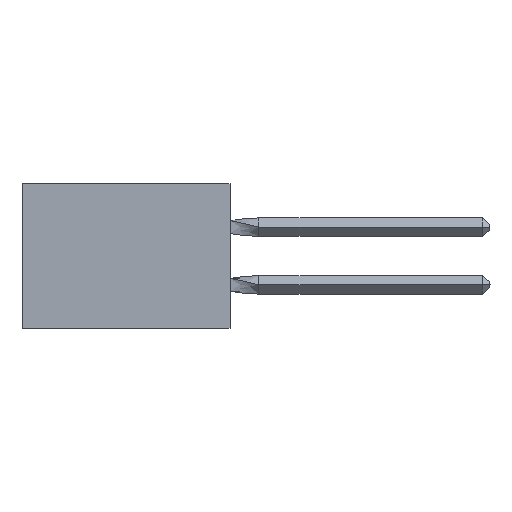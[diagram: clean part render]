
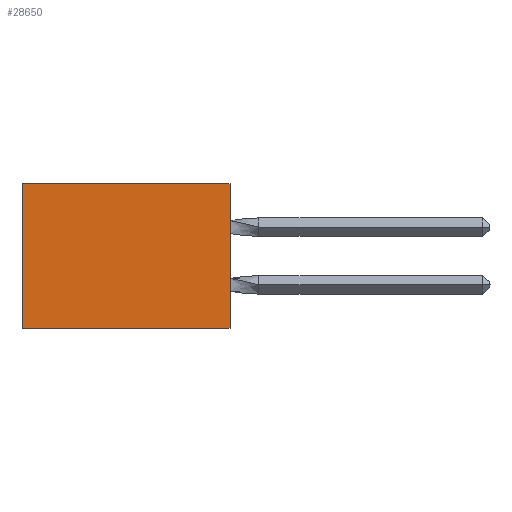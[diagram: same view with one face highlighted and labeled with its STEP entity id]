
A CAD part, left-side view. The second image highlights one B-rep face of the part: STEP entity #28650.
In plain terms, the highlighted planar face has unit normal (-1, 0, 0).
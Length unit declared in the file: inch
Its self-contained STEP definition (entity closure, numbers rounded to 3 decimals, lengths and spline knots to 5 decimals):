
#1717 = DIRECTION ( 'NONE',  ( 0., 0., -1. ) ) ;
#2243 = VERTEX_POINT ( 'NONE', #22399 ) ;
#3325 = FACE_OUTER_BOUND ( 'NONE', #24013, .T. ) ;
#3617 = DIRECTION ( 'NONE',  ( 0., 1., 0. ) ) ;
#7488 = CARTESIAN_POINT ( 'NONE',  ( 0.305, 0.72, 0. ) ) ;
#8642 = ORIENTED_EDGE ( 'NONE', *, *, #11522, .F. ) ;
#9768 = CARTESIAN_POINT ( 'NONE',  ( 0.305, 0., -0.5 ) ) ;
#10783 = DIRECTION ( 'NONE',  ( 0., 0., -1. ) ) ;
#11522 = EDGE_CURVE ( 'NONE', #2243, #32752, #19938, .T. ) ;
#13785 = VECTOR ( 'NONE', #28690, 39.37008 ) ;
#14025 = EDGE_CURVE ( 'NONE', #37685, #32752, #37899, .T. ) ;
#19022 = CARTESIAN_POINT ( 'NONE',  ( 0.305, 0., -0.5 ) ) ;
#19802 = DIRECTION ( 'NONE',  ( 0., 1., 0. ) ) ;
#19938 = LINE ( 'NONE', #19022, #22840 ) ;
#22052 = CARTESIAN_POINT ( 'NONE',  ( 0.305, 0.72, -0.5 ) ) ;
#22165 = ORIENTED_EDGE ( 'NONE', *, *, #38047, .T. ) ;
#22399 = CARTESIAN_POINT ( 'NONE',  ( 0.305, 0., -0.5 ) ) ;
#22832 = ORIENTED_EDGE ( 'NONE', *, *, #14025, .T. ) ;
#22840 = VECTOR ( 'NONE', #3617, 39.37008 ) ;
#23538 = PLANE ( 'NONE',  #28241 ) ;
#23675 = DIRECTION ( 'NONE',  ( 1., 0., 0. ) ) ;
#24013 = EDGE_LOOP ( 'NONE', ( #22832, #8642, #32874, #22165 ) ) ;
#25680 = VERTEX_POINT ( 'NONE', #35800 ) ;
#28241 = AXIS2_PLACEMENT_3D ( 'NONE', #39223, #23675, #1717 ) ;
#28650 = ADVANCED_FACE ( 'NONE', ( #3325 ), #23538, .F. ) ;
#28690 = DIRECTION ( 'NONE',  ( 0., 0., -1. ) ) ;
#32605 = CARTESIAN_POINT ( 'NONE',  ( 0.305, 0.72, -0.5 ) ) ;
#32752 = VERTEX_POINT ( 'NONE', #22052 ) ;
#32874 = ORIENTED_EDGE ( 'NONE', *, *, #33789, .F. ) ;
#33789 = EDGE_CURVE ( 'NONE', #25680, #2243, #39344, .T. ) ;
#34706 = LINE ( 'NONE', #38299, #40112 ) ;
#35800 = CARTESIAN_POINT ( 'NONE',  ( 0.305, 0., 0. ) ) ;
#36919 = VECTOR ( 'NONE', #10783, 39.37008 ) ;
#37685 = VERTEX_POINT ( 'NONE', #7488 ) ;
#37899 = LINE ( 'NONE', #32605, #36919 ) ;
#38047 = EDGE_CURVE ( 'NONE', #25680, #37685, #34706, .T. ) ;
#38299 = CARTESIAN_POINT ( 'NONE',  ( 0.305, 0., 0. ) ) ;
#39223 = CARTESIAN_POINT ( 'NONE',  ( 0.305, 0., -0.5 ) ) ;
#39344 = LINE ( 'NONE', #9768, #13785 ) ;
#40112 = VECTOR ( 'NONE', #19802, 39.37008 ) ;
